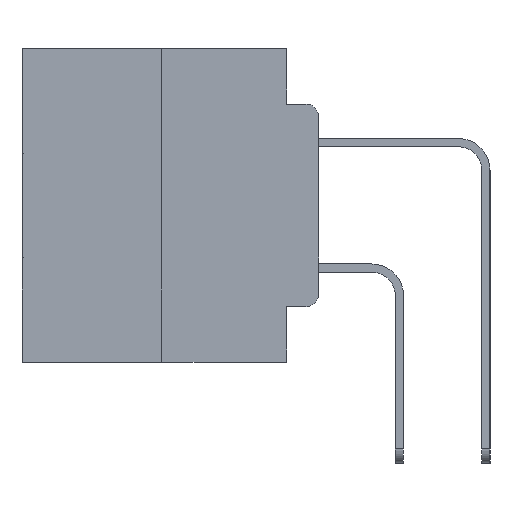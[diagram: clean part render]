
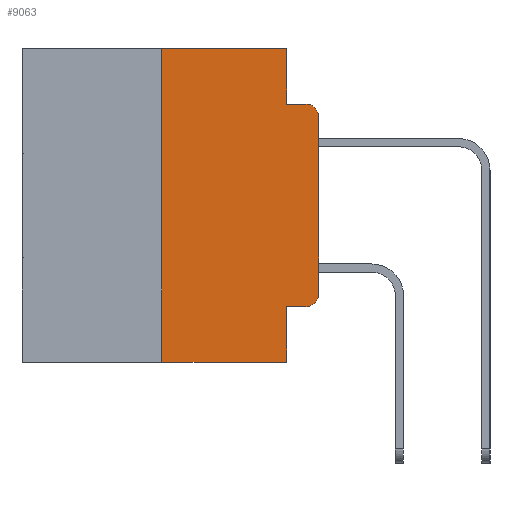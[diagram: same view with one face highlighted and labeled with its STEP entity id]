
A CAD part, left-side view. The second image highlights one B-rep face of the part: STEP entity #9063.
In plain terms, the highlighted planar face has unit normal (-1, 0, 0).
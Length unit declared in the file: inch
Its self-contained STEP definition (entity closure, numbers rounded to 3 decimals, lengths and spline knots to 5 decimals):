
#135 = CARTESIAN_POINT ( 'NONE',  ( 0., 0., 0. ) ) ;
#464 = VERTEX_POINT ( 'NONE', #12723 ) ;
#587 = VERTEX_POINT ( 'NONE', #17570 ) ;
#1065 = VERTEX_POINT ( 'NONE', #10624 ) ;
#1382 = CARTESIAN_POINT ( 'NONE',  ( 0., 0.051, 0. ) ) ;
#1405 = ORIENTED_EDGE ( 'NONE', *, *, #11743, .T. ) ;
#1703 = CARTESIAN_POINT ( 'NONE',  ( 0., 0.02, -0.3915 ) ) ;
#2037 = DIRECTION ( 'NONE',  ( 0., 0., 1. ) ) ;
#2166 = EDGE_LOOP ( 'NONE', ( #9834, #4174, #22939, #17645, #24307, #6798, #4908, #18015, #29855, #1405 ) ) ;
#2244 = VECTOR ( 'NONE', #25357, 39.37008 ) ;
#4174 = ORIENTED_EDGE ( 'NONE', *, *, #28336, .T. ) ;
#4220 = DIRECTION ( 'NONE',  ( 0., 0., -1. ) ) ;
#4790 = EDGE_CURVE ( 'NONE', #16878, #14749, #10928, .T. ) ;
#4835 = DIRECTION ( 'NONE',  ( -1., 0., 0. ) ) ;
#4908 = ORIENTED_EDGE ( 'NONE', *, *, #10021, .T. ) ;
#5681 = AXIS2_PLACEMENT_3D ( 'NONE', #1703, #18181, #4220 ) ;
#6049 = LINE ( 'NONE', #28335, #16956 ) ;
#6200 = VECTOR ( 'NONE', #27507, 39.37008 ) ;
#6489 = DIRECTION ( 'NONE',  ( 1., 0., 0. ) ) ;
#6625 = LINE ( 'NONE', #23881, #24162 ) ;
#6798 = ORIENTED_EDGE ( 'NONE', *, *, #20891, .F. ) ;
#7080 = CARTESIAN_POINT ( 'NONE',  ( 0., 0.051, 0. ) ) ;
#7238 = VERTEX_POINT ( 'NONE', #12173 ) ;
#9063 = ADVANCED_FACE ( 'NONE', ( #12354 ), #15735, .F. ) ;
#9510 = DIRECTION ( 'NONE',  ( 0., 0., -1. ) ) ;
#9834 = ORIENTED_EDGE ( 'NONE', *, *, #4790, .T. ) ;
#10017 = CARTESIAN_POINT ( 'NONE',  ( 0., 0.473, 0. ) ) ;
#10021 = EDGE_CURVE ( 'NONE', #1065, #587, #6049, .T. ) ;
#10610 = CARTESIAN_POINT ( 'NONE',  ( 0., 0.051, -0.4115 ) ) ;
#10624 = CARTESIAN_POINT ( 'NONE',  ( 0., 0.25, -0.5 ) ) ;
#10928 = LINE ( 'NONE', #135, #22295 ) ;
#11112 = VERTEX_POINT ( 'NONE', #26631 ) ;
#11378 = EDGE_CURVE ( 'NONE', #7238, #464, #28754, .T. ) ;
#11584 = AXIS2_PLACEMENT_3D ( 'NONE', #18760, #4835, #21022 ) ;
#11717 = CARTESIAN_POINT ( 'NONE',  ( 0., 0.051, -0.4115 ) ) ;
#11743 = EDGE_CURVE ( 'NONE', #11112, #16878, #13622, .T. ) ;
#11929 = CARTESIAN_POINT ( 'NONE',  ( 0., 0.25, 0. ) ) ;
#12173 = CARTESIAN_POINT ( 'NONE',  ( 0., 0.25, 0. ) ) ;
#12354 = FACE_OUTER_BOUND ( 'NONE', #2166, .T. ) ;
#12588 = DIRECTION ( 'NONE',  ( 0., -1., 0. ) ) ;
#12723 = CARTESIAN_POINT ( 'NONE',  ( 0., 0.051, 0. ) ) ;
#12752 = VERTEX_POINT ( 'NONE', #21590 ) ;
#13415 = DIRECTION ( 'NONE',  ( 0., 0., -1. ) ) ;
#13622 = CIRCLE ( 'NONE', #5681, 0.02 ) ;
#14547 = CIRCLE ( 'NONE', #11584, 0.02 ) ;
#14749 = VERTEX_POINT ( 'NONE', #20192 ) ;
#14835 = LINE ( 'NONE', #11929, #2244 ) ;
#15735 = PLANE ( 'NONE',  #24794 ) ;
#16647 = VECTOR ( 'NONE', #13415, 39.37008 ) ;
#16878 = VERTEX_POINT ( 'NONE', #24030 ) ;
#16956 = VECTOR ( 'NONE', #12588, 39.37008 ) ;
#17268 = LINE ( 'NONE', #7080, #29319 ) ;
#17570 = CARTESIAN_POINT ( 'NONE',  ( 0., 0.051, -0.5 ) ) ;
#17645 = ORIENTED_EDGE ( 'NONE', *, *, #25368, .F. ) ;
#17849 = EDGE_CURVE ( 'NONE', #26969, #11112, #28978, .T. ) ;
#18015 = ORIENTED_EDGE ( 'NONE', *, *, #19370, .F. ) ;
#18181 = DIRECTION ( 'NONE',  ( -1., 0., 0. ) ) ;
#18760 = CARTESIAN_POINT ( 'NONE',  ( 0., 0.02, -0.1085 ) ) ;
#19370 = EDGE_CURVE ( 'NONE', #26969, #587, #29906, .T. ) ;
#19378 = DIRECTION ( 'NONE',  ( 0., -1., 0. ) ) ;
#20192 = CARTESIAN_POINT ( 'NONE',  ( 0., 0., -0.1085 ) ) ;
#20891 = EDGE_CURVE ( 'NONE', #1065, #7238, #14835, .T. ) ;
#21022 = DIRECTION ( 'NONE',  ( 0., 0., -1. ) ) ;
#21590 = CARTESIAN_POINT ( 'NONE',  ( 0., 0.051, -0.0885 ) ) ;
#22120 = VERTEX_POINT ( 'NONE', #28989 ) ;
#22295 = VECTOR ( 'NONE', #2037, 39.37008 ) ;
#22568 = DIRECTION ( 'NONE',  ( 0., 0., -1. ) ) ;
#22939 = ORIENTED_EDGE ( 'NONE', *, *, #26881, .F. ) ;
#23606 = DIRECTION ( 'NONE',  ( 0., -1., 0. ) ) ;
#23881 = CARTESIAN_POINT ( 'NONE',  ( 0., 0.051, -0.0885 ) ) ;
#24030 = CARTESIAN_POINT ( 'NONE',  ( 0., 0., -0.3915 ) ) ;
#24162 = VECTOR ( 'NONE', #19378, 39.37008 ) ;
#24307 = ORIENTED_EDGE ( 'NONE', *, *, #11378, .F. ) ;
#24794 = AXIS2_PLACEMENT_3D ( 'NONE', #29053, #6489, #22568 ) ;
#25357 = DIRECTION ( 'NONE',  ( 0., 0., 1. ) ) ;
#25368 = EDGE_CURVE ( 'NONE', #464, #12752, #17268, .T. ) ;
#26631 = CARTESIAN_POINT ( 'NONE',  ( 0., 0.02, -0.4115 ) ) ;
#26881 = EDGE_CURVE ( 'NONE', #12752, #22120, #6625, .T. ) ;
#26969 = VERTEX_POINT ( 'NONE', #10610 ) ;
#27507 = DIRECTION ( 'NONE',  ( 0., -1., 0. ) ) ;
#28335 = CARTESIAN_POINT ( 'NONE',  ( 0., 0.473, -0.5 ) ) ;
#28336 = EDGE_CURVE ( 'NONE', #14749, #22120, #14547, .T. ) ;
#28754 = LINE ( 'NONE', #10017, #29436 ) ;
#28978 = LINE ( 'NONE', #11717, #6200 ) ;
#28989 = CARTESIAN_POINT ( 'NONE',  ( 0., 0.02, -0.0885 ) ) ;
#29053 = CARTESIAN_POINT ( 'NONE',  ( 0., 0.473, 0. ) ) ;
#29319 = VECTOR ( 'NONE', #9510, 39.37008 ) ;
#29436 = VECTOR ( 'NONE', #23606, 39.37008 ) ;
#29855 = ORIENTED_EDGE ( 'NONE', *, *, #17849, .T. ) ;
#29906 = LINE ( 'NONE', #1382, #16647 ) ;
